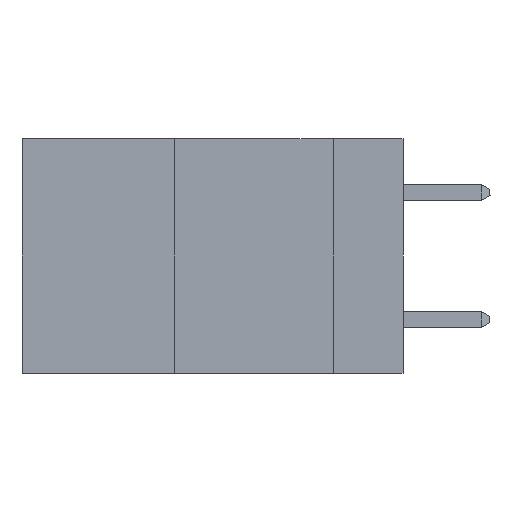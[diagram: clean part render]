
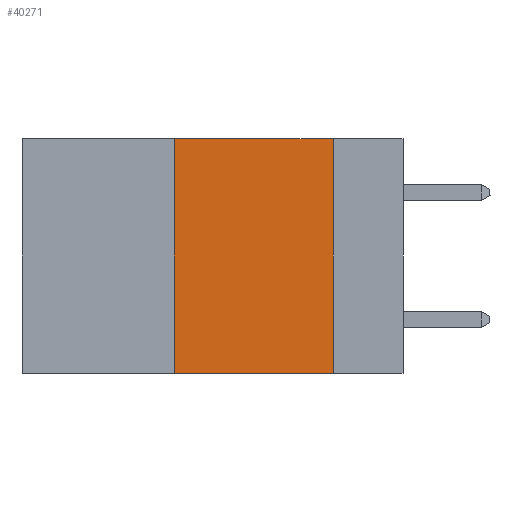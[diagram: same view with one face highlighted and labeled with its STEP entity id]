
A CAD part, left-side view. The second image highlights one B-rep face of the part: STEP entity #40271.
In plain terms, the highlighted planar face has unit normal (-1, 0, 0).
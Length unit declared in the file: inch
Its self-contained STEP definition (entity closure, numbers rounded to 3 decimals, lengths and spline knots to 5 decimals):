
#183 = CARTESIAN_POINT ( 'NONE',  ( 0., 0.36, 0. ) ) ;
#1536 = CARTESIAN_POINT ( 'NONE',  ( 0., 0.6, 0. ) ) ;
#2967 = VERTEX_POINT ( 'NONE', #7128 ) ;
#5295 = ORIENTED_EDGE ( 'NONE', *, *, #38151, .F. ) ;
#6027 = ORIENTED_EDGE ( 'NONE', *, *, #31114, .T. ) ;
#6196 = EDGE_CURVE ( 'NONE', #32914, #30884, #22374, .T. ) ;
#6244 = CARTESIAN_POINT ( 'NONE',  ( 0., 0.36, -0.37 ) ) ;
#7128 = CARTESIAN_POINT ( 'NONE',  ( 0., 0.36, 0. ) ) ;
#8471 = DIRECTION ( 'NONE',  ( 1., 0., 0. ) ) ;
#11167 = DIRECTION ( 'NONE',  ( 0., -1., 0. ) ) ;
#11396 = CARTESIAN_POINT ( 'NONE',  ( 0., 0.11, -0.37 ) ) ;
#12031 = FACE_OUTER_BOUND ( 'NONE', #24343, .T. ) ;
#13160 = DIRECTION ( 'NONE',  ( 0., 0., 1. ) ) ;
#14781 = EDGE_CURVE ( 'NONE', #2967, #32914, #17677, .T. ) ;
#14987 = ORIENTED_EDGE ( 'NONE', *, *, #6196, .F. ) ;
#15354 = VECTOR ( 'NONE', #13160, 39.37008 ) ;
#17677 = LINE ( 'NONE', #1536, #24667 ) ;
#20338 = CARTESIAN_POINT ( 'NONE',  ( 0., 0.6, -0.37 ) ) ;
#21430 = VERTEX_POINT ( 'NONE', #6244 ) ;
#22374 = LINE ( 'NONE', #29661, #32400 ) ;
#23470 = LINE ( 'NONE', #20338, #28894 ) ;
#24343 = EDGE_LOOP ( 'NONE', ( #14987, #37310, #5295, #6027 ) ) ;
#24667 = VECTOR ( 'NONE', #11167, 39.37008 ) ;
#25927 = LINE ( 'NONE', #183, #15354 ) ;
#26490 = AXIS2_PLACEMENT_3D ( 'NONE', #27936, #8471, #37787 ) ;
#26804 = DIRECTION ( 'NONE',  ( 0., -1., 0. ) ) ;
#27936 = CARTESIAN_POINT ( 'NONE',  ( 0., 0.6, 0. ) ) ;
#28839 = DIRECTION ( 'NONE',  ( 0., 0., -1. ) ) ;
#28894 = VECTOR ( 'NONE', #26804, 39.37008 ) ;
#29661 = CARTESIAN_POINT ( 'NONE',  ( 0., 0.11, 0. ) ) ;
#30884 = VERTEX_POINT ( 'NONE', #11396 ) ;
#31114 = EDGE_CURVE ( 'NONE', #21430, #30884, #23470, .T. ) ;
#32400 = VECTOR ( 'NONE', #28839, 39.37008 ) ;
#32914 = VERTEX_POINT ( 'NONE', #37936 ) ;
#34027 = PLANE ( 'NONE',  #26490 ) ;
#37310 = ORIENTED_EDGE ( 'NONE', *, *, #14781, .F. ) ;
#37787 = DIRECTION ( 'NONE',  ( 0., 0., -1. ) ) ;
#37936 = CARTESIAN_POINT ( 'NONE',  ( 0., 0.11, 0. ) ) ;
#38151 = EDGE_CURVE ( 'NONE', #21430, #2967, #25927, .T. ) ;
#40271 = ADVANCED_FACE ( 'NONE', ( #12031 ), #34027, .F. ) ;
